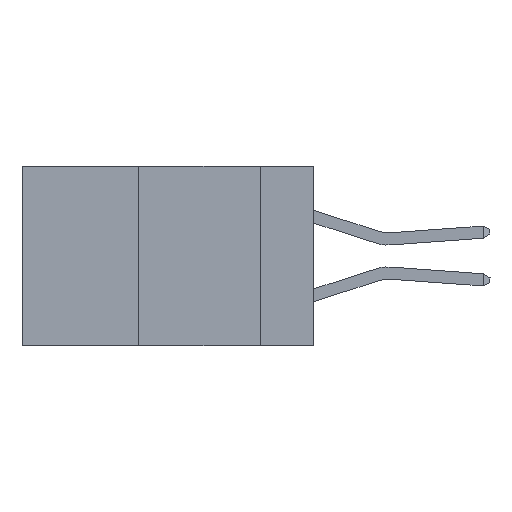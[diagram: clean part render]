
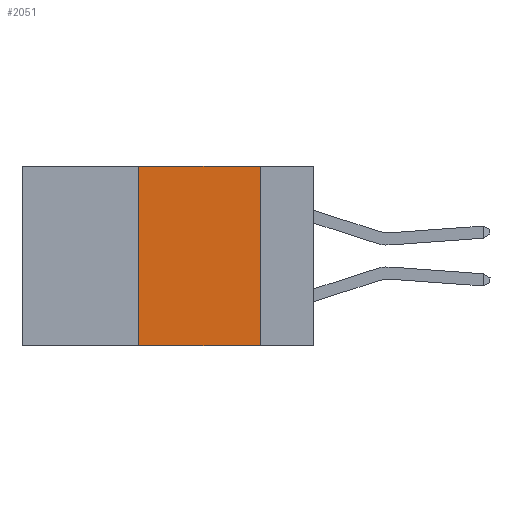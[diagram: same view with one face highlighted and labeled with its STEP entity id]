
A CAD part, left-side view. The second image highlights one B-rep face of the part: STEP entity #2051.
In plain terms, the highlighted planar face has unit normal (-1, 0, 0).
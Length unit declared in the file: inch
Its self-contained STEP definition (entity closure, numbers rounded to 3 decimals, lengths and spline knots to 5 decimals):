
#1745 = VERTEX_POINT ( 'NONE', #15188 ) ;
#2042 = CARTESIAN_POINT ( 'NONE',  ( 0., 0.36, 0. ) ) ;
#2051 = ADVANCED_FACE ( 'NONE', ( #19662 ), #18101, .F. ) ;
#2202 = CARTESIAN_POINT ( 'NONE',  ( 0., 0.6, -0.37 ) ) ;
#2689 = ORIENTED_EDGE ( 'NONE', *, *, #6623, .F. ) ;
#3642 = CARTESIAN_POINT ( 'NONE',  ( 0., 0.11, 0. ) ) ;
#4189 = DIRECTION ( 'NONE',  ( 0., -1., 0. ) ) ;
#6421 = DIRECTION ( 'NONE',  ( 0., 0., -1. ) ) ;
#6623 = EDGE_CURVE ( 'NONE', #12336, #18742, #19070, .T. ) ;
#7223 = ORIENTED_EDGE ( 'NONE', *, *, #24675, .F. ) ;
#8122 = EDGE_CURVE ( 'NONE', #23908, #1745, #16584, .T. ) ;
#8600 = DIRECTION ( 'NONE',  ( 1., 0., 0. ) ) ;
#8751 = VECTOR ( 'NONE', #21345, 39.37008 ) ;
#8767 = ORIENTED_EDGE ( 'NONE', *, *, #8122, .F. ) ;
#10112 = DIRECTION ( 'NONE',  ( 0., 0., -1. ) ) ;
#11877 = CARTESIAN_POINT ( 'NONE',  ( 0., 0.6, 0. ) ) ;
#11913 = EDGE_LOOP ( 'NONE', ( #2689, #7223, #8767, #14710 ) ) ;
#12334 = VECTOR ( 'NONE', #4189, 39.37008 ) ;
#12336 = VERTEX_POINT ( 'NONE', #3642 ) ;
#14200 = AXIS2_PLACEMENT_3D ( 'NONE', #21714, #8600, #10112 ) ;
#14710 = ORIENTED_EDGE ( 'NONE', *, *, #24699, .T. ) ;
#14819 = CARTESIAN_POINT ( 'NONE',  ( 0., 0.36, -0.37 ) ) ;
#15188 = CARTESIAN_POINT ( 'NONE',  ( 0., 0.36, 0. ) ) ;
#16584 = LINE ( 'NONE', #2042, #23775 ) ;
#17880 = CARTESIAN_POINT ( 'NONE',  ( 0., 0.11, 0. ) ) ;
#18101 = PLANE ( 'NONE',  #14200 ) ;
#18742 = VERTEX_POINT ( 'NONE', #21819 ) ;
#19070 = LINE ( 'NONE', #17880, #20550 ) ;
#19662 = FACE_OUTER_BOUND ( 'NONE', #11913, .T. ) ;
#19800 = LINE ( 'NONE', #2202, #8751 ) ;
#20550 = VECTOR ( 'NONE', #6421, 39.37008 ) ;
#20760 = DIRECTION ( 'NONE',  ( 0., 0., 1. ) ) ;
#21345 = DIRECTION ( 'NONE',  ( 0., -1., 0. ) ) ;
#21714 = CARTESIAN_POINT ( 'NONE',  ( 0., 0.6, 0. ) ) ;
#21819 = CARTESIAN_POINT ( 'NONE',  ( 0., 0.11, -0.37 ) ) ;
#22493 = LINE ( 'NONE', #11877, #12334 ) ;
#23775 = VECTOR ( 'NONE', #20760, 39.37008 ) ;
#23908 = VERTEX_POINT ( 'NONE', #14819 ) ;
#24675 = EDGE_CURVE ( 'NONE', #1745, #12336, #22493, .T. ) ;
#24699 = EDGE_CURVE ( 'NONE', #23908, #18742, #19800, .T. ) ;
